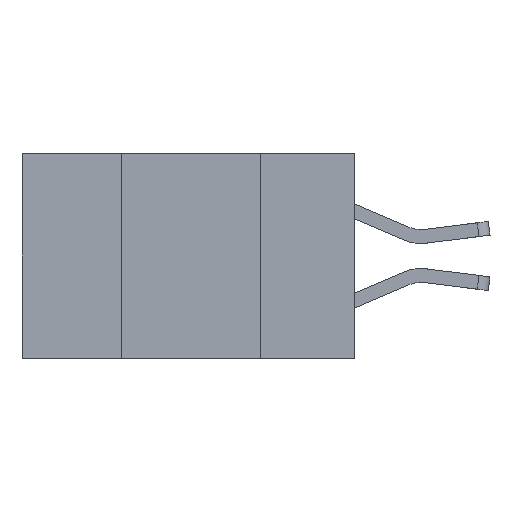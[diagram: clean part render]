
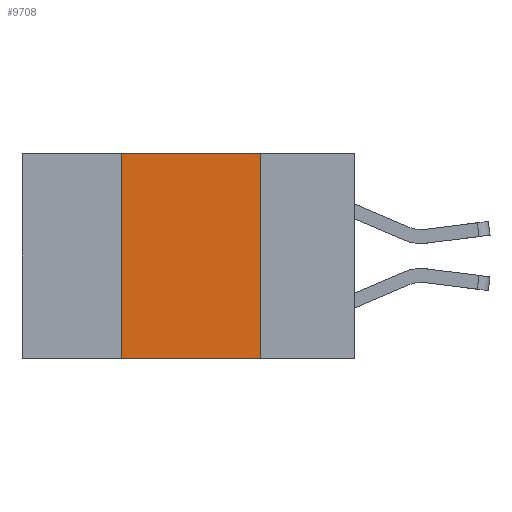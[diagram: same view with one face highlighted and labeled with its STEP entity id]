
A CAD part, left-side view. The second image highlights one B-rep face of the part: STEP entity #9708.
In plain terms, the highlighted planar face has unit normal (-1, 0, 0).
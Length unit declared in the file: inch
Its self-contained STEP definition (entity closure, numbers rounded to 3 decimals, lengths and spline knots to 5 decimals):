
#215 = VECTOR ( 'NONE', #7832, 39.37008 ) ;
#234 = ORIENTED_EDGE ( 'NONE', *, *, #7997, .F. ) ;
#352 = PLANE ( 'NONE',  #631 ) ;
#631 = AXIS2_PLACEMENT_3D ( 'NONE', #2442, #9335, #3460 ) ;
#637 = DIRECTION ( 'NONE',  ( 0., 0., -1. ) ) ;
#845 = LINE ( 'NONE', #12013, #5983 ) ;
#850 = EDGE_LOOP ( 'NONE', ( #234, #2856, #6807, #2708 ) ) ;
#1861 = VECTOR ( 'NONE', #10618, 39.37008 ) ;
#2442 = CARTESIAN_POINT ( 'NONE',  ( 0., 0.6, 0. ) ) ;
#2708 = ORIENTED_EDGE ( 'NONE', *, *, #8011, .T. ) ;
#2856 = ORIENTED_EDGE ( 'NONE', *, *, #7686, .F. ) ;
#3119 = FACE_OUTER_BOUND ( 'NONE', #850, .T. ) ;
#3269 = LINE ( 'NONE', #9579, #5677 ) ;
#3460 = DIRECTION ( 'NONE',  ( 0., 0., -1. ) ) ;
#3934 = VERTEX_POINT ( 'NONE', #8263 ) ;
#5080 = VERTEX_POINT ( 'NONE', #7474 ) ;
#5116 = VERTEX_POINT ( 'NONE', #8546 ) ;
#5677 = VECTOR ( 'NONE', #7791, 39.37008 ) ;
#5983 = VECTOR ( 'NONE', #637, 39.37008 ) ;
#6807 = ORIENTED_EDGE ( 'NONE', *, *, #8009, .F. ) ;
#6827 = CARTESIAN_POINT ( 'NONE',  ( 0., 0.6, -0.37 ) ) ;
#7474 = CARTESIAN_POINT ( 'NONE',  ( 0., 0.42, -0.37 ) ) ;
#7686 = EDGE_CURVE ( 'NONE', #5116, #8366, #10478, .T. ) ;
#7791 = DIRECTION ( 'NONE',  ( 0., 0., 1. ) ) ;
#7832 = DIRECTION ( 'NONE',  ( 0., -1., 0. ) ) ;
#7997 = EDGE_CURVE ( 'NONE', #8366, #3934, #845, .T. ) ;
#8009 = EDGE_CURVE ( 'NONE', #5080, #5116, #3269, .T. ) ;
#8011 = EDGE_CURVE ( 'NONE', #5080, #3934, #8347, .T. ) ;
#8263 = CARTESIAN_POINT ( 'NONE',  ( 0., 0.17, -0.37 ) ) ;
#8347 = LINE ( 'NONE', #6827, #215 ) ;
#8366 = VERTEX_POINT ( 'NONE', #11897 ) ;
#8546 = CARTESIAN_POINT ( 'NONE',  ( 0., 0.42, 0. ) ) ;
#9335 = DIRECTION ( 'NONE',  ( 1., 0., 0. ) ) ;
#9579 = CARTESIAN_POINT ( 'NONE',  ( 0., 0.42, 0. ) ) ;
#9708 = ADVANCED_FACE ( 'NONE', ( #3119 ), #352, .F. ) ;
#10478 = LINE ( 'NONE', #12199, #1861 ) ;
#10618 = DIRECTION ( 'NONE',  ( 0., -1., 0. ) ) ;
#11897 = CARTESIAN_POINT ( 'NONE',  ( 0., 0.17, 0. ) ) ;
#12013 = CARTESIAN_POINT ( 'NONE',  ( 0., 0.17, 0. ) ) ;
#12199 = CARTESIAN_POINT ( 'NONE',  ( 0., 0.6, 0. ) ) ;
